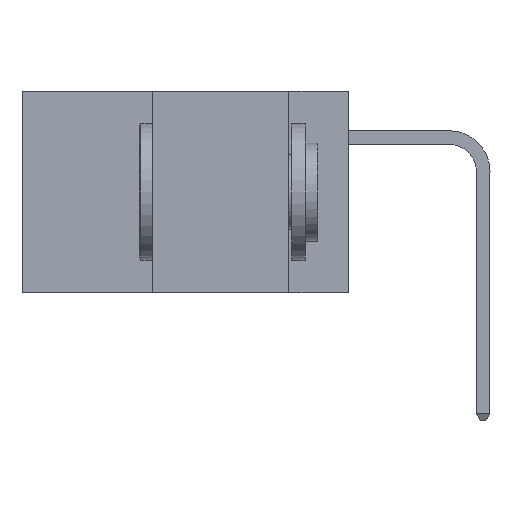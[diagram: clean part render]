
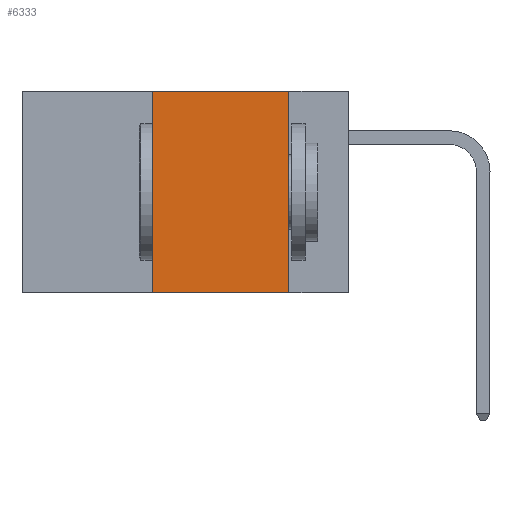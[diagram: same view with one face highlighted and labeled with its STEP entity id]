
A CAD part, left-side view. The second image highlights one B-rep face of the part: STEP entity #6333.
In plain terms, the highlighted planar face has unit normal (-1, 0, 0).
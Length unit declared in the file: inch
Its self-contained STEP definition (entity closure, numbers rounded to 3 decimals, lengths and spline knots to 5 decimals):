
#13 = DIRECTION ( 'NONE',  ( 0., -1., 0. ) ) ;
#89 = FACE_OUTER_BOUND ( 'NONE', #7928, .T. ) ;
#879 = VERTEX_POINT ( 'NONE', #7292 ) ;
#1218 = VERTEX_POINT ( 'NONE', #12892 ) ;
#2189 = VECTOR ( 'NONE', #3452, 39.37008 ) ;
#2306 = CARTESIAN_POINT ( 'NONE',  ( 0., 0.11, -0.37 ) ) ;
#2692 = PLANE ( 'NONE',  #12914 ) ;
#3452 = DIRECTION ( 'NONE',  ( 0., 0., 1. ) ) ;
#3737 = DIRECTION ( 'NONE',  ( 0., 0., -1. ) ) ;
#4907 = CARTESIAN_POINT ( 'NONE',  ( 0., 0.11, 0. ) ) ;
#5193 = ORIENTED_EDGE ( 'NONE', *, *, #6438, .F. ) ;
#5300 = VECTOR ( 'NONE', #12025, 39.37008 ) ;
#5729 = EDGE_CURVE ( 'NONE', #8560, #1218, #11163, .T. ) ;
#5755 = ORIENTED_EDGE ( 'NONE', *, *, #5729, .F. ) ;
#5889 = CARTESIAN_POINT ( 'NONE',  ( 0., 0.36, 0. ) ) ;
#6068 = ORIENTED_EDGE ( 'NONE', *, *, #11701, .F. ) ;
#6248 = ORIENTED_EDGE ( 'NONE', *, *, #12294, .T. ) ;
#6333 = ADVANCED_FACE ( 'NONE', ( #89 ), #2692, .F. ) ;
#6438 = EDGE_CURVE ( 'NONE', #1218, #13060, #11006, .T. ) ;
#7292 = CARTESIAN_POINT ( 'NONE',  ( 0., 0.36, -0.37 ) ) ;
#7542 = CARTESIAN_POINT ( 'NONE',  ( 0., 0.6, -0.37 ) ) ;
#7751 = CARTESIAN_POINT ( 'NONE',  ( 0., 0.36, 0. ) ) ;
#7864 = LINE ( 'NONE', #7751, #2189 ) ;
#7928 = EDGE_LOOP ( 'NONE', ( #5193, #5755, #6068, #6248 ) ) ;
#8045 = CARTESIAN_POINT ( 'NONE',  ( 0., 0.6, 0. ) ) ;
#8560 = VERTEX_POINT ( 'NONE', #5889 ) ;
#9320 = VECTOR ( 'NONE', #13, 39.37008 ) ;
#10084 = DIRECTION ( 'NONE',  ( 1., 0., 0. ) ) ;
#11006 = LINE ( 'NONE', #4907, #12297 ) ;
#11009 = CARTESIAN_POINT ( 'NONE',  ( 0., 0.6, 0. ) ) ;
#11163 = LINE ( 'NONE', #8045, #5300 ) ;
#11701 = EDGE_CURVE ( 'NONE', #879, #8560, #7864, .T. ) ;
#11890 = LINE ( 'NONE', #7542, #9320 ) ;
#12025 = DIRECTION ( 'NONE',  ( 0., -1., 0. ) ) ;
#12294 = EDGE_CURVE ( 'NONE', #879, #13060, #11890, .T. ) ;
#12297 = VECTOR ( 'NONE', #12991, 39.37008 ) ;
#12892 = CARTESIAN_POINT ( 'NONE',  ( 0., 0.11, 0. ) ) ;
#12914 = AXIS2_PLACEMENT_3D ( 'NONE', #11009, #10084, #3737 ) ;
#12991 = DIRECTION ( 'NONE',  ( 0., 0., -1. ) ) ;
#13060 = VERTEX_POINT ( 'NONE', #2306 ) ;
